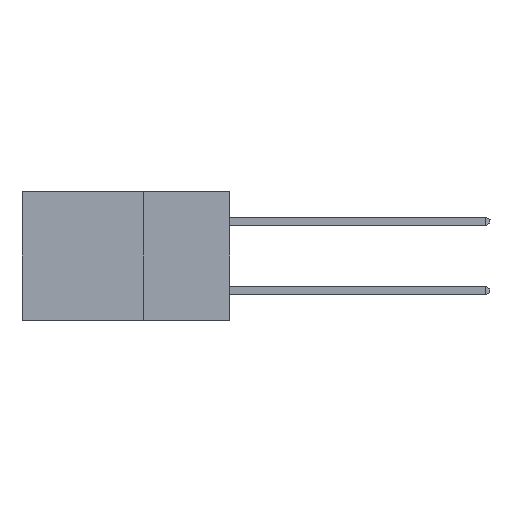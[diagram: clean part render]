
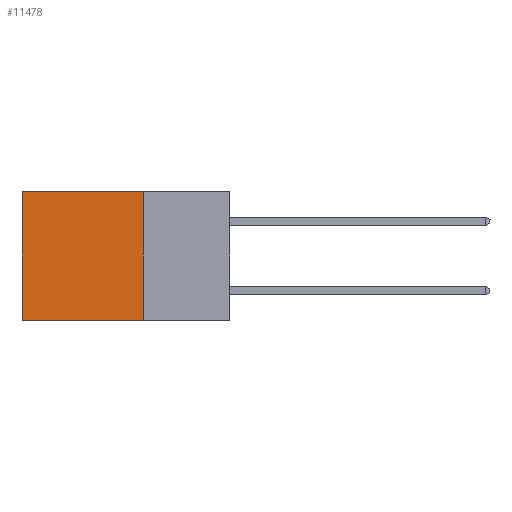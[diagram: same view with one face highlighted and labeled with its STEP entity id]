
A CAD part, left-side view. The second image highlights one B-rep face of the part: STEP entity #11478.
In plain terms, the highlighted planar face has unit normal (-1, 0, 0).
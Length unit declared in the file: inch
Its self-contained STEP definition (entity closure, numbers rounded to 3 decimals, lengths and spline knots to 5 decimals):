
#161 = VERTEX_POINT ( 'NONE', #506 ) ;
#238 = LINE ( 'NONE', #9570, #4514 ) ;
#266 = ORIENTED_EDGE ( 'NONE', *, *, #4419, .F. ) ;
#506 = CARTESIAN_POINT ( 'NONE',  ( 0.298, 0.6, -0.37 ) ) ;
#667 = FACE_OUTER_BOUND ( 'NONE', #10967, .T. ) ;
#973 = DIRECTION ( 'NONE',  ( 0., 0., -1. ) ) ;
#1183 = EDGE_CURVE ( 'NONE', #2622, #161, #5852, .T. ) ;
#1485 = DIRECTION ( 'NONE',  ( 0., 0., -1. ) ) ;
#1704 = AXIS2_PLACEMENT_3D ( 'NONE', #2576, #11781, #7134 ) ;
#2187 = CARTESIAN_POINT ( 'NONE',  ( 0.298, 0.25, -0.37 ) ) ;
#2216 = VECTOR ( 'NONE', #973, 39.37008 ) ;
#2576 = CARTESIAN_POINT ( 'NONE',  ( 0.298, 0.25, 0. ) ) ;
#2622 = VERTEX_POINT ( 'NONE', #4837 ) ;
#2755 = CARTESIAN_POINT ( 'NONE',  ( 0.298, 0.25, -0.37 ) ) ;
#3503 = ORIENTED_EDGE ( 'NONE', *, *, #7762, .F. ) ;
#4106 = VECTOR ( 'NONE', #7243, 39.37008 ) ;
#4419 = EDGE_CURVE ( 'NONE', #7571, #6282, #7084, .T. ) ;
#4514 = VECTOR ( 'NONE', #9532, 39.37008 ) ;
#4837 = CARTESIAN_POINT ( 'NONE',  ( 0.298, 0.6, 0. ) ) ;
#5183 = CARTESIAN_POINT ( 'NONE',  ( 0.298, 0.6, 0. ) ) ;
#5240 = LINE ( 'NONE', #2755, #4106 ) ;
#5479 = CARTESIAN_POINT ( 'NONE',  ( 0.298, 0.25, 0. ) ) ;
#5852 = LINE ( 'NONE', #5183, #9227 ) ;
#6282 = VERTEX_POINT ( 'NONE', #2187 ) ;
#6823 = ORIENTED_EDGE ( 'NONE', *, *, #8089, .T. ) ;
#7084 = LINE ( 'NONE', #5479, #2216 ) ;
#7134 = DIRECTION ( 'NONE',  ( 0., 0., -1. ) ) ;
#7243 = DIRECTION ( 'NONE',  ( 0., 1., 0. ) ) ;
#7571 = VERTEX_POINT ( 'NONE', #11332 ) ;
#7762 = EDGE_CURVE ( 'NONE', #6282, #161, #5240, .T. ) ;
#8089 = EDGE_CURVE ( 'NONE', #7571, #2622, #238, .T. ) ;
#9227 = VECTOR ( 'NONE', #1485, 39.37008 ) ;
#9532 = DIRECTION ( 'NONE',  ( 0., 1., 0. ) ) ;
#9570 = CARTESIAN_POINT ( 'NONE',  ( 0.298, 0.25, 0. ) ) ;
#10469 = ORIENTED_EDGE ( 'NONE', *, *, #1183, .T. ) ;
#10967 = EDGE_LOOP ( 'NONE', ( #10469, #3503, #266, #6823 ) ) ;
#11332 = CARTESIAN_POINT ( 'NONE',  ( 0.298, 0.25, 0. ) ) ;
#11478 = ADVANCED_FACE ( 'NONE', ( #667 ), #11698, .F. ) ;
#11698 = PLANE ( 'NONE',  #1704 ) ;
#11781 = DIRECTION ( 'NONE',  ( 1., 0., 0. ) ) ;
